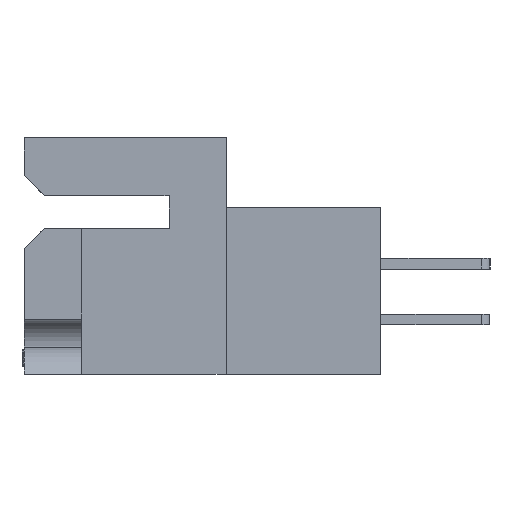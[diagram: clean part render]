
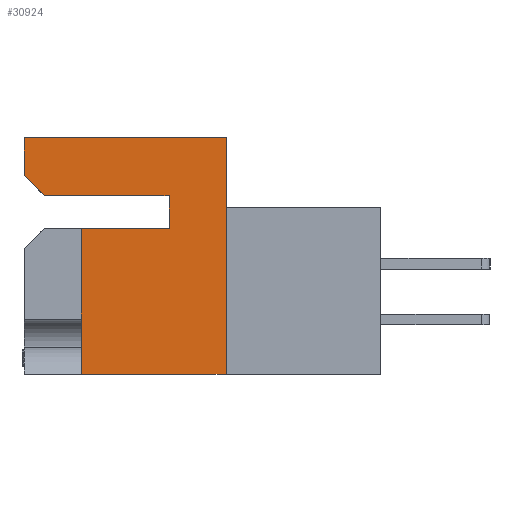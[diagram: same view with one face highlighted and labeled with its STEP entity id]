
A CAD part, left-side view. The second image highlights one B-rep face of the part: STEP entity #30924.
In plain terms, the highlighted planar face has unit normal (-1, 0, 0).
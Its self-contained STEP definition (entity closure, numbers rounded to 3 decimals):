
#698 = VERTEX_POINT ( 'NONE', #909 ) ;
#909 = CARTESIAN_POINT ( 'NONE',  ( 0., 11.506, -2.159 ) ) ;
#1450 = ORIENTED_EDGE ( 'NONE', *, *, #17340, .F. ) ;
#1499 = DIRECTION ( 'NONE',  ( 0., 0., -1. ) ) ;
#1877 = VERTEX_POINT ( 'NONE', #16033 ) ;
#3120 = EDGE_CURVE ( 'NONE', #30999, #12727, #33653, .T. ) ;
#3853 = ORIENTED_EDGE ( 'NONE', *, *, #11416, .F. ) ;
#4189 = CARTESIAN_POINT ( 'NONE',  ( 0., 10.363, -3.302 ) ) ;
#4467 = ORIENTED_EDGE ( 'NONE', *, *, #26927, .F. ) ;
#6856 = VERTEX_POINT ( 'NONE', #14602 ) ;
#7347 = PLANE ( 'NONE',  #22251 ) ;
#7424 = EDGE_CURVE ( 'NONE', #698, #6856, #28398, .T. ) ;
#7559 = LINE ( 'NONE', #18882, #10936 ) ;
#7578 = VECTOR ( 'NONE', #17412, 1000. ) ;
#7932 = DIRECTION ( 'NONE',  ( 0., 0., -1. ) ) ;
#8426 = CARTESIAN_POINT ( 'NONE',  ( 0., 8.255, -5.182 ) ) ;
#8596 = CARTESIAN_POINT ( 'NONE',  ( 0., -8.814, -13.487 ) ) ;
#8814 = EDGE_CURVE ( 'NONE', #698, #20199, #11253, .T. ) ;
#9049 = ORIENTED_EDGE ( 'NONE', *, *, #30490, .F. ) ;
#9206 = CARTESIAN_POINT ( 'NONE',  ( 0., 3.251, -3.302 ) ) ;
#9391 = DIRECTION ( 'NONE',  ( 0., -0.707, -0.707 ) ) ;
#9623 = CARTESIAN_POINT ( 'NONE',  ( 0., 0., -13.487 ) ) ;
#10196 = CARTESIAN_POINT ( 'NONE',  ( 0., 11.506, 0. ) ) ;
#10936 = VECTOR ( 'NONE', #7932, 1000. ) ;
#11253 = LINE ( 'NONE', #19064, #17658 ) ;
#11416 = EDGE_CURVE ( 'NONE', #14750, #29482, #19606, .T. ) ;
#11423 = VECTOR ( 'NONE', #30427, 1000. ) ;
#12664 = LINE ( 'NONE', #14268, #13561 ) ;
#12727 = VERTEX_POINT ( 'NONE', #9206 ) ;
#13561 = VECTOR ( 'NONE', #22344, 1000. ) ;
#13783 = DIRECTION ( 'NONE',  ( 0., 1., 0. ) ) ;
#14268 = CARTESIAN_POINT ( 'NONE',  ( 0., 8.255, -5.182 ) ) ;
#14602 = CARTESIAN_POINT ( 'NONE',  ( 0., 10.363, -3.302 ) ) ;
#14750 = VERTEX_POINT ( 'NONE', #9623 ) ;
#14811 = LINE ( 'NONE', #28404, #7578 ) ;
#14946 = VECTOR ( 'NONE', #13783, 1000. ) ;
#16033 = CARTESIAN_POINT ( 'NONE',  ( 0., 0., 0. ) ) ;
#17340 = EDGE_CURVE ( 'NONE', #29482, #35188, #12664, .T. ) ;
#17412 = DIRECTION ( 'NONE',  ( 0., 1., 0. ) ) ;
#17658 = VECTOR ( 'NONE', #21816, 1000. ) ;
#17786 = DIRECTION ( 'NONE',  ( 1., 0., 0. ) ) ;
#17830 = VECTOR ( 'NONE', #20932, 1000. ) ;
#17851 = EDGE_CURVE ( 'NONE', #35188, #30999, #24187, .T. ) ;
#18882 = CARTESIAN_POINT ( 'NONE',  ( 0., 0., 0. ) ) ;
#19064 = CARTESIAN_POINT ( 'NONE',  ( 0., 11.506, -13.487 ) ) ;
#19285 = CARTESIAN_POINT ( 'NONE',  ( 0., 0., -5.182 ) ) ;
#19606 = LINE ( 'NONE', #8596, #14946 ) ;
#20199 = VERTEX_POINT ( 'NONE', #21088 ) ;
#20290 = ORIENTED_EDGE ( 'NONE', *, *, #7424, .T. ) ;
#20932 = DIRECTION ( 'NONE',  ( 0., -1., 0. ) ) ;
#21088 = CARTESIAN_POINT ( 'NONE',  ( 0., 11.506, 0. ) ) ;
#21514 = VECTOR ( 'NONE', #9391, 1000. ) ;
#21816 = DIRECTION ( 'NONE',  ( 0., 0., 1. ) ) ;
#22022 = DIRECTION ( 'NONE',  ( 0., -1., 0. ) ) ;
#22173 = ORIENTED_EDGE ( 'NONE', *, *, #3120, .F. ) ;
#22251 = AXIS2_PLACEMENT_3D ( 'NONE', #34310, #17786, #1499 ) ;
#22344 = DIRECTION ( 'NONE',  ( 0., 0., 1. ) ) ;
#22529 = ORIENTED_EDGE ( 'NONE', *, *, #17851, .F. ) ;
#24134 = CARTESIAN_POINT ( 'NONE',  ( 0., 3.251, -5.182 ) ) ;
#24187 = LINE ( 'NONE', #19285, #29777 ) ;
#24666 = ORIENTED_EDGE ( 'NONE', *, *, #8814, .F. ) ;
#25242 = CARTESIAN_POINT ( 'NONE',  ( 0., 3.251, -5.182 ) ) ;
#26746 = FACE_OUTER_BOUND ( 'NONE', #34244, .T. ) ;
#26927 = EDGE_CURVE ( 'NONE', #20199, #1877, #29839, .T. ) ;
#27214 = CARTESIAN_POINT ( 'NONE',  ( 0., 8.255, -13.487 ) ) ;
#27393 = EDGE_CURVE ( 'NONE', #12727, #6856, #14811, .T. ) ;
#28398 = LINE ( 'NONE', #4189, #21514 ) ;
#28404 = CARTESIAN_POINT ( 'NONE',  ( 0., 0., -3.302 ) ) ;
#28702 = ORIENTED_EDGE ( 'NONE', *, *, #27393, .F. ) ;
#29482 = VERTEX_POINT ( 'NONE', #27214 ) ;
#29777 = VECTOR ( 'NONE', #22022, 1000. ) ;
#29839 = LINE ( 'NONE', #10196, #17830 ) ;
#30427 = DIRECTION ( 'NONE',  ( 0., 0., 1. ) ) ;
#30490 = EDGE_CURVE ( 'NONE', #1877, #14750, #7559, .T. ) ;
#30924 = ADVANCED_FACE ( 'NONE', ( #26746 ), #7347, .F. ) ;
#30999 = VERTEX_POINT ( 'NONE', #24134 ) ;
#33653 = LINE ( 'NONE', #25242, #11423 ) ;
#34244 = EDGE_LOOP ( 'NONE', ( #3853, #9049, #4467, #24666, #20290, #28702, #22173, #22529, #1450 ) ) ;
#34310 = CARTESIAN_POINT ( 'NONE',  ( 0., 0., 0. ) ) ;
#35188 = VERTEX_POINT ( 'NONE', #8426 ) ;
